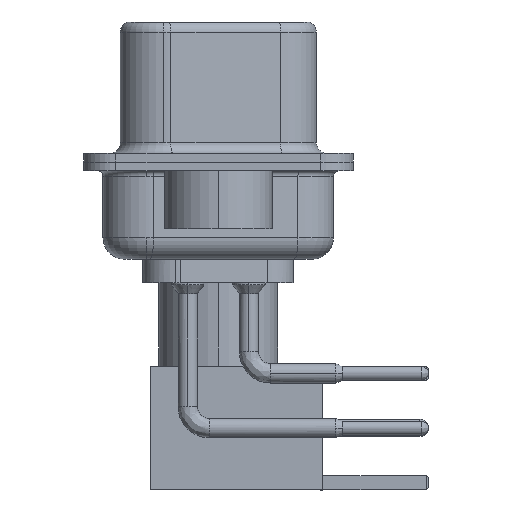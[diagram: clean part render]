
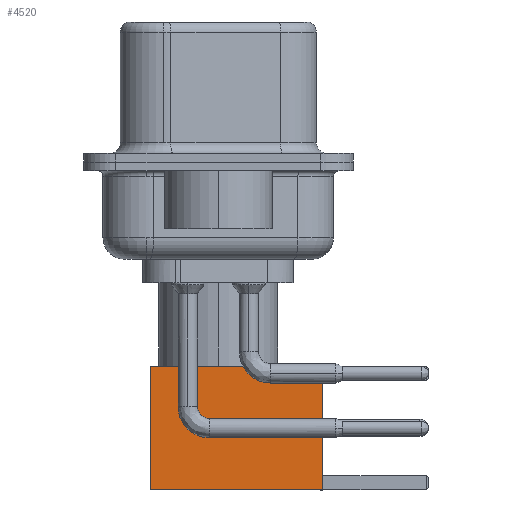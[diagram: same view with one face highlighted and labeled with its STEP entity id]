
A CAD part, left-side view. The second image highlights one B-rep face of the part: STEP entity #4520.
In plain terms, the highlighted face is planar.
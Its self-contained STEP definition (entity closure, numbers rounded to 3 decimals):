
#681 = LINE ( 'NONE', #10219, #7998 ) ;
#978 = VERTEX_POINT ( 'NONE', #10213 ) ;
#2333 = FACE_OUTER_BOUND ( 'NONE', #10154, .T. ) ;
#3034 = ORIENTED_EDGE ( 'NONE', *, *, #14690, .F. ) ;
#3770 = VECTOR ( 'NONE', #23711, 1000. ) ;
#4479 = DIRECTION ( 'NONE',  ( 0., 1., 0. ) ) ;
#4520 = ADVANCED_FACE ( 'NONE', ( #2333 ), #25284, .T. ) ;
#5292 = ORIENTED_EDGE ( 'NONE', *, *, #17574, .T. ) ;
#6358 = LINE ( 'NONE', #14470, #16135 ) ;
#6593 = CARTESIAN_POINT ( 'NONE',  ( -2.875, 2.875, 0. ) ) ;
#7998 = VECTOR ( 'NONE', #20219, 1000. ) ;
#10154 = EDGE_LOOP ( 'NONE', ( #5292, #17382, #22763, #3034 ) ) ;
#10213 = CARTESIAN_POINT ( 'NONE',  ( 2.875, 2.875, 8. ) ) ;
#10219 = CARTESIAN_POINT ( 'NONE',  ( -2.875, 2.875, 0. ) ) ;
#10513 = CARTESIAN_POINT ( 'NONE',  ( 0., 2.875, 8. ) ) ;
#12739 = CARTESIAN_POINT ( 'NONE',  ( 2.875, 2.875, 0. ) ) ;
#12892 = DIRECTION ( 'NONE',  ( -1., 0., 0. ) ) ;
#13691 = CARTESIAN_POINT ( 'NONE',  ( 2.875, 2.875, 0. ) ) ;
#13934 = VERTEX_POINT ( 'NONE', #20871 ) ;
#14470 = CARTESIAN_POINT ( 'NONE',  ( 0., 2.875, 0. ) ) ;
#14690 = EDGE_CURVE ( 'NONE', #978, #19781, #22782, .T. ) ;
#16135 = VECTOR ( 'NONE', #21671, 1000. ) ;
#16860 = VECTOR ( 'NONE', #12892, 1000. ) ;
#17382 = ORIENTED_EDGE ( 'NONE', *, *, #17934, .T. ) ;
#17574 = EDGE_CURVE ( 'NONE', #978, #13934, #17702, .T. ) ;
#17702 = LINE ( 'NONE', #13691, #3770 ) ;
#17934 = EDGE_CURVE ( 'NONE', #13934, #24569, #6358, .T. ) ;
#18782 = AXIS2_PLACEMENT_3D ( 'NONE', #12739, #4479, #18881 ) ;
#18881 = DIRECTION ( 'NONE',  ( 0., 0., 1. ) ) ;
#19781 = VERTEX_POINT ( 'NONE', #25034 ) ;
#20219 = DIRECTION ( 'NONE',  ( 0., 0., -1. ) ) ;
#20871 = CARTESIAN_POINT ( 'NONE',  ( 2.875, 2.875, 0. ) ) ;
#21671 = DIRECTION ( 'NONE',  ( -1., 0., 0. ) ) ;
#22763 = ORIENTED_EDGE ( 'NONE', *, *, #26334, .F. ) ;
#22782 = LINE ( 'NONE', #10513, #16860 ) ;
#23711 = DIRECTION ( 'NONE',  ( 0., 0., -1. ) ) ;
#24569 = VERTEX_POINT ( 'NONE', #6593 ) ;
#25034 = CARTESIAN_POINT ( 'NONE',  ( -2.875, 2.875, 8. ) ) ;
#25284 = PLANE ( 'NONE',  #18782 ) ;
#26334 = EDGE_CURVE ( 'NONE', #19781, #24569, #681, .T. ) ;
